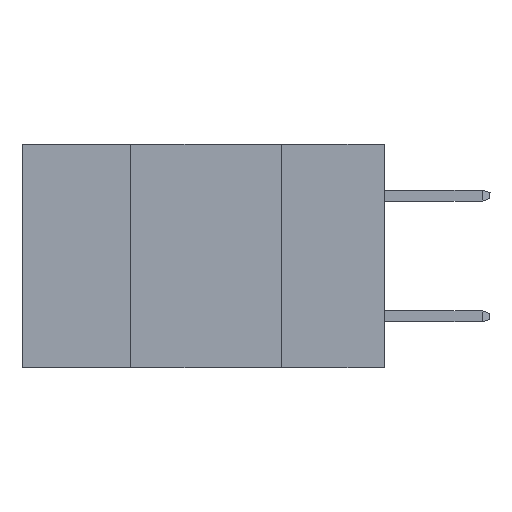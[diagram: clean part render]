
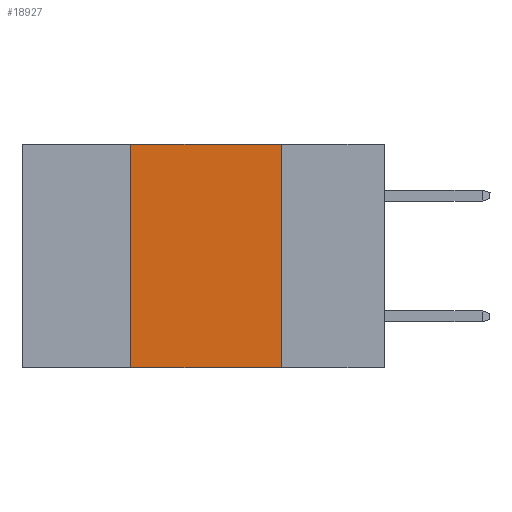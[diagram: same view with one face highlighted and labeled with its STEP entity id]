
A CAD part, left-side view. The second image highlights one B-rep face of the part: STEP entity #18927.
In plain terms, the highlighted planar face has unit normal (-1, 0, 0).
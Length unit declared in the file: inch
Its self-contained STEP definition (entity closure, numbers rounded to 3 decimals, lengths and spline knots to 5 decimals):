
#128 = VECTOR ( 'NONE', #18975, 39.37008 ) ;
#522 = CARTESIAN_POINT ( 'NONE',  ( 0., 0.6, 0. ) ) ;
#586 = LINE ( 'NONE', #522, #9589 ) ;
#1826 = EDGE_CURVE ( 'NONE', #6263, #4127, #14326, .T. ) ;
#2152 = DIRECTION ( 'NONE',  ( 0., -1., 0. ) ) ;
#2710 = VERTEX_POINT ( 'NONE', #11370 ) ;
#3731 = EDGE_CURVE ( 'NONE', #2710, #6263, #586, .T. ) ;
#4127 = VERTEX_POINT ( 'NONE', #25463 ) ;
#6263 = VERTEX_POINT ( 'NONE', #24409 ) ;
#7304 = VECTOR ( 'NONE', #10721, 39.37008 ) ;
#8218 = EDGE_CURVE ( 'NONE', #21991, #4127, #23435, .T. ) ;
#8222 = EDGE_LOOP ( 'NONE', ( #23556, #11775, #24317, #19014 ) ) ;
#8343 = CARTESIAN_POINT ( 'NONE',  ( 0., 0.6, 0. ) ) ;
#9516 = EDGE_CURVE ( 'NONE', #21991, #2710, #20236, .T. ) ;
#9589 = VECTOR ( 'NONE', #2152, 39.37008 ) ;
#10643 = CARTESIAN_POINT ( 'NONE',  ( 0., 0.6, -0.37 ) ) ;
#10721 = DIRECTION ( 'NONE',  ( 0., -1., 0. ) ) ;
#11370 = CARTESIAN_POINT ( 'NONE',  ( 0., 0.42, 0. ) ) ;
#11775 = ORIENTED_EDGE ( 'NONE', *, *, #3731, .F. ) ;
#12524 = DIRECTION ( 'NONE',  ( 0., 0., -1. ) ) ;
#12947 = CARTESIAN_POINT ( 'NONE',  ( 0., 0.42, -0.37 ) ) ;
#14316 = DIRECTION ( 'NONE',  ( 1., 0., 0. ) ) ;
#14326 = LINE ( 'NONE', #24381, #16519 ) ;
#14569 = PLANE ( 'NONE',  #21141 ) ;
#16519 = VECTOR ( 'NONE', #24023, 39.37008 ) ;
#18103 = FACE_OUTER_BOUND ( 'NONE', #8222, .T. ) ;
#18927 = ADVANCED_FACE ( 'NONE', ( #18103 ), #14569, .F. ) ;
#18975 = DIRECTION ( 'NONE',  ( 0., 0., 1. ) ) ;
#19014 = ORIENTED_EDGE ( 'NONE', *, *, #8218, .T. ) ;
#20236 = LINE ( 'NONE', #22824, #128 ) ;
#21141 = AXIS2_PLACEMENT_3D ( 'NONE', #8343, #14316, #12524 ) ;
#21991 = VERTEX_POINT ( 'NONE', #12947 ) ;
#22824 = CARTESIAN_POINT ( 'NONE',  ( 0., 0.42, 0. ) ) ;
#23435 = LINE ( 'NONE', #10643, #7304 ) ;
#23556 = ORIENTED_EDGE ( 'NONE', *, *, #1826, .F. ) ;
#24023 = DIRECTION ( 'NONE',  ( 0., 0., -1. ) ) ;
#24317 = ORIENTED_EDGE ( 'NONE', *, *, #9516, .F. ) ;
#24381 = CARTESIAN_POINT ( 'NONE',  ( 0., 0.17, 0. ) ) ;
#24409 = CARTESIAN_POINT ( 'NONE',  ( 0., 0.17, 0. ) ) ;
#25463 = CARTESIAN_POINT ( 'NONE',  ( 0., 0.17, -0.37 ) ) ;
